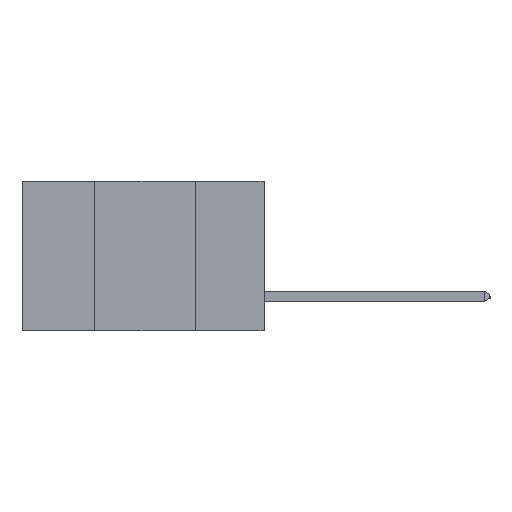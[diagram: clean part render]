
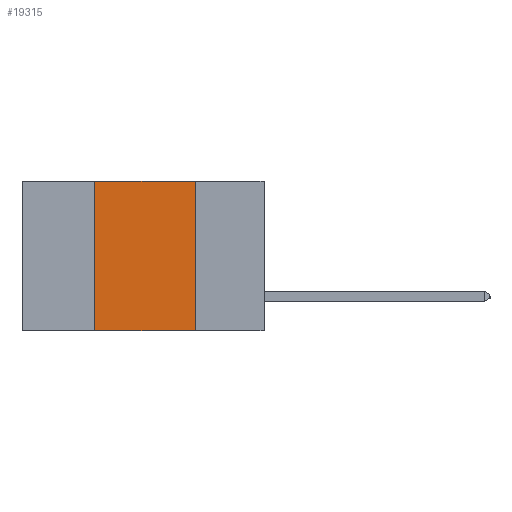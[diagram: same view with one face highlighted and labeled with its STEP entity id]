
A CAD part, left-side view. The second image highlights one B-rep face of the part: STEP entity #19315.
In plain terms, the highlighted planar face has unit normal (-1, 0, 0).
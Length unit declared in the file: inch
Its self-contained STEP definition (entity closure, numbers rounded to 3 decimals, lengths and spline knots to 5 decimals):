
#59 = DIRECTION ( 'NONE',  ( 0., 0., -1. ) ) ;
#1061 = CARTESIAN_POINT ( 'NONE',  ( 0., 0.17, 0. ) ) ;
#1147 = DIRECTION ( 'NONE',  ( 0., 0., -1. ) ) ;
#1148 = EDGE_CURVE ( 'NONE', #4280, #2975, #5476, .T. ) ;
#2094 = LINE ( 'NONE', #4234, #11497 ) ;
#2391 = EDGE_CURVE ( 'NONE', #4280, #4741, #2411, .T. ) ;
#2411 = LINE ( 'NONE', #21450, #11790 ) ;
#2655 = EDGE_CURVE ( 'NONE', #4741, #11426, #2094, .T. ) ;
#2975 = VERTEX_POINT ( 'NONE', #7433 ) ;
#3942 = AXIS2_PLACEMENT_3D ( 'NONE', #18559, #11359, #59 ) ;
#3969 = ORIENTED_EDGE ( 'NONE', *, *, #1148, .T. ) ;
#4141 = LINE ( 'NONE', #1061, #8536 ) ;
#4234 = CARTESIAN_POINT ( 'NONE',  ( 0., 0.6, 0. ) ) ;
#4280 = VERTEX_POINT ( 'NONE', #23981 ) ;
#4741 = VERTEX_POINT ( 'NONE', #15443 ) ;
#4949 = EDGE_CURVE ( 'NONE', #11426, #2975, #4141, .T. ) ;
#5476 = LINE ( 'NONE', #18529, #19529 ) ;
#7433 = CARTESIAN_POINT ( 'NONE',  ( 0., 0.17, -0.37 ) ) ;
#8536 = VECTOR ( 'NONE', #1147, 39.37008 ) ;
#9524 = ORIENTED_EDGE ( 'NONE', *, *, #4949, .F. ) ;
#10305 = DIRECTION ( 'NONE',  ( 0., 0., 1. ) ) ;
#11359 = DIRECTION ( 'NONE',  ( 1., 0., 0. ) ) ;
#11426 = VERTEX_POINT ( 'NONE', #16667 ) ;
#11497 = VECTOR ( 'NONE', #14557, 39.37008 ) ;
#11790 = VECTOR ( 'NONE', #10305, 39.37008 ) ;
#14557 = DIRECTION ( 'NONE',  ( 0., -1., 0. ) ) ;
#15443 = CARTESIAN_POINT ( 'NONE',  ( 0., 0.42, 0. ) ) ;
#16116 = EDGE_LOOP ( 'NONE', ( #9524, #19801, #23504, #3969 ) ) ;
#16667 = CARTESIAN_POINT ( 'NONE',  ( 0., 0.17, 0. ) ) ;
#16893 = DIRECTION ( 'NONE',  ( 0., -1., 0. ) ) ;
#18529 = CARTESIAN_POINT ( 'NONE',  ( 0., 0.6, -0.37 ) ) ;
#18559 = CARTESIAN_POINT ( 'NONE',  ( 0., 0.6, 0. ) ) ;
#19315 = ADVANCED_FACE ( 'NONE', ( #19945 ), #22251, .F. ) ;
#19529 = VECTOR ( 'NONE', #16893, 39.37008 ) ;
#19801 = ORIENTED_EDGE ( 'NONE', *, *, #2655, .F. ) ;
#19945 = FACE_OUTER_BOUND ( 'NONE', #16116, .T. ) ;
#21450 = CARTESIAN_POINT ( 'NONE',  ( 0., 0.42, 0. ) ) ;
#22251 = PLANE ( 'NONE',  #3942 ) ;
#23504 = ORIENTED_EDGE ( 'NONE', *, *, #2391, .F. ) ;
#23981 = CARTESIAN_POINT ( 'NONE',  ( 0., 0.42, -0.37 ) ) ;
